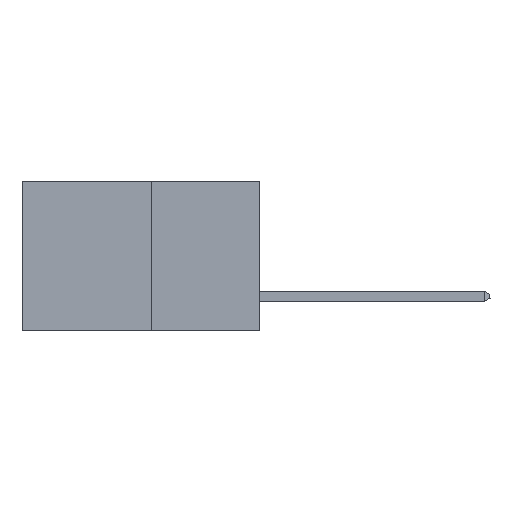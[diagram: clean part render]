
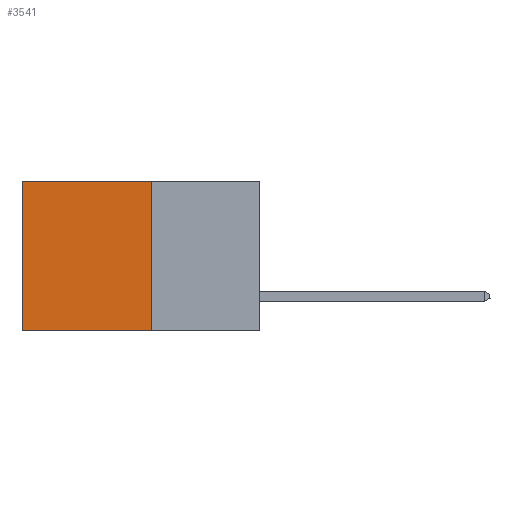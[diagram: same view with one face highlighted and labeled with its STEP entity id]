
A CAD part, left-side view. The second image highlights one B-rep face of the part: STEP entity #3541.
In plain terms, the highlighted planar face has unit normal (-1, 0, 0).
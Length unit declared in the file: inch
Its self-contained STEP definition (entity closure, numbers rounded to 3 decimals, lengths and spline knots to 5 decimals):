
#669 = DIRECTION ( 'NONE',  ( 0., 1., 0. ) ) ;
#1535 = DIRECTION ( 'NONE',  ( 0., 0., -1. ) ) ;
#1591 = CARTESIAN_POINT ( 'NONE',  ( 0.277, 0.27, -0.37 ) ) ;
#2085 = VECTOR ( 'NONE', #669, 39.37008 ) ;
#2532 = LINE ( 'NONE', #3509, #2085 ) ;
#3000 = PLANE ( 'NONE',  #10745 ) ;
#3481 = VERTEX_POINT ( 'NONE', #14928 ) ;
#3489 = VECTOR ( 'NONE', #1535, 39.37008 ) ;
#3509 = CARTESIAN_POINT ( 'NONE',  ( 0.277, 0.27, 0. ) ) ;
#3541 = ADVANCED_FACE ( 'NONE', ( #13292 ), #3000, .F. ) ;
#3951 = LINE ( 'NONE', #8601, #3489 ) ;
#4599 = DIRECTION ( 'NONE',  ( 0., 0., -1. ) ) ;
#5002 = ORIENTED_EDGE ( 'NONE', *, *, #9118, .T. ) ;
#5529 = VERTEX_POINT ( 'NONE', #10792 ) ;
#6012 = VERTEX_POINT ( 'NONE', #6558 ) ;
#6558 = CARTESIAN_POINT ( 'NONE',  ( 0.277, 0.59, 0. ) ) ;
#6559 = DIRECTION ( 'NONE',  ( 0., 1., 0. ) ) ;
#7326 = VECTOR ( 'NONE', #15842, 39.37008 ) ;
#7730 = CARTESIAN_POINT ( 'NONE',  ( 0.277, 0.59, -0.37 ) ) ;
#7882 = EDGE_CURVE ( 'NONE', #11414, #5529, #13350, .T. ) ;
#8601 = CARTESIAN_POINT ( 'NONE',  ( 0.277, 0.27, -0.37 ) ) ;
#9118 = EDGE_CURVE ( 'NONE', #6012, #5529, #14134, .T. ) ;
#9565 = EDGE_CURVE ( 'NONE', #3481, #11414, #3951, .T. ) ;
#10745 = AXIS2_PLACEMENT_3D ( 'NONE', #1591, #11260, #4599 ) ;
#10792 = CARTESIAN_POINT ( 'NONE',  ( 0.277, 0.59, -0.37 ) ) ;
#11260 = DIRECTION ( 'NONE',  ( 1., 0., 0. ) ) ;
#11414 = VERTEX_POINT ( 'NONE', #12597 ) ;
#12047 = EDGE_LOOP ( 'NONE', ( #5002, #14653, #14973, #12656 ) ) ;
#12597 = CARTESIAN_POINT ( 'NONE',  ( 0.277, 0.27, -0.37 ) ) ;
#12656 = ORIENTED_EDGE ( 'NONE', *, *, #16581, .T. ) ;
#12932 = VECTOR ( 'NONE', #6559, 39.37008 ) ;
#13292 = FACE_OUTER_BOUND ( 'NONE', #12047, .T. ) ;
#13350 = LINE ( 'NONE', #15998, #12932 ) ;
#14134 = LINE ( 'NONE', #7730, #7326 ) ;
#14653 = ORIENTED_EDGE ( 'NONE', *, *, #7882, .F. ) ;
#14928 = CARTESIAN_POINT ( 'NONE',  ( 0.277, 0.27, 0. ) ) ;
#14973 = ORIENTED_EDGE ( 'NONE', *, *, #9565, .F. ) ;
#15842 = DIRECTION ( 'NONE',  ( 0., 0., -1. ) ) ;
#15998 = CARTESIAN_POINT ( 'NONE',  ( 0.277, 0.27, -0.37 ) ) ;
#16581 = EDGE_CURVE ( 'NONE', #3481, #6012, #2532, .T. ) ;
